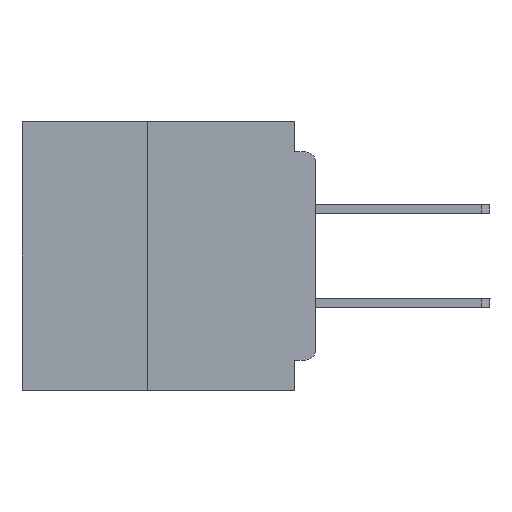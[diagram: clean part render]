
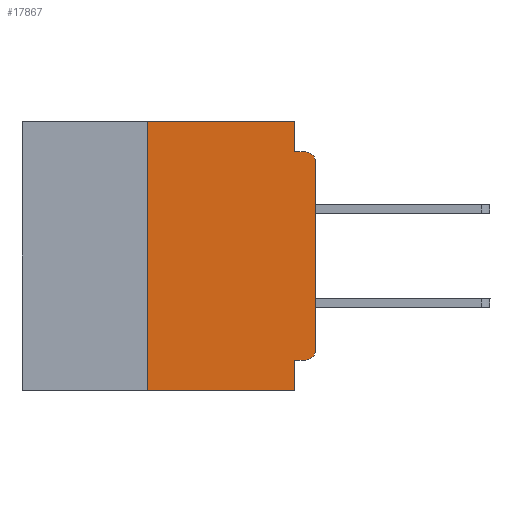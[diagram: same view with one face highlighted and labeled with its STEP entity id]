
A CAD part, left-side view. The second image highlights one B-rep face of the part: STEP entity #17867.
In plain terms, the highlighted planar face has unit normal (-1, 0, 0).
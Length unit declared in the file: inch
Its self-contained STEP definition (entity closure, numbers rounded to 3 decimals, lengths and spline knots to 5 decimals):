
#1379 = VECTOR ( 'NONE', #47287, 39.37008 ) ;
#3993 = CARTESIAN_POINT ( 'NONE',  ( 0., 0., 0. ) ) ;
#5181 = LINE ( 'NONE', #22048, #29538 ) ;
#7249 = VERTEX_POINT ( 'NONE', #17080 ) ;
#7311 = ORIENTED_EDGE ( 'NONE', *, *, #21296, .F. ) ;
#8545 = VERTEX_POINT ( 'NONE', #12974 ) ;
#9433 = VERTEX_POINT ( 'NONE', #9885 ) ;
#9720 = CARTESIAN_POINT ( 'NONE',  ( 0., 0.031, -0.355 ) ) ;
#9763 = ORIENTED_EDGE ( 'NONE', *, *, #60409, .T. ) ;
#9885 = CARTESIAN_POINT ( 'NONE',  ( 0., 0.031, -0.045 ) ) ;
#11398 = CARTESIAN_POINT ( 'NONE',  ( 0., 0., -0.34 ) ) ;
#12096 = DIRECTION ( 'NONE',  ( 0., -1., 0. ) ) ;
#12740 = CARTESIAN_POINT ( 'NONE',  ( 0., 0.031, 0. ) ) ;
#12939 = DIRECTION ( 'NONE',  ( -1., 0., 0. ) ) ;
#12974 = CARTESIAN_POINT ( 'NONE',  ( 0., 0.031, -0.4 ) ) ;
#13891 = VERTEX_POINT ( 'NONE', #11398 ) ;
#13942 = EDGE_CURVE ( 'NONE', #17463, #8545, #29659, .T. ) ;
#14390 = LINE ( 'NONE', #51946, #1379 ) ;
#16096 = PLANE ( 'NONE',  #57764 ) ;
#16668 = CARTESIAN_POINT ( 'NONE',  ( 0., 0.437, -0.4 ) ) ;
#17066 = CARTESIAN_POINT ( 'NONE',  ( 0., 0.015, -0.34 ) ) ;
#17080 = CARTESIAN_POINT ( 'NONE',  ( 0., 0.25, 0. ) ) ;
#17463 = VERTEX_POINT ( 'NONE', #61303 ) ;
#17867 = ADVANCED_FACE ( 'NONE', ( #32133 ), #16096, .F. ) ;
#17999 = DIRECTION ( 'NONE',  ( 0., 0., -1. ) ) ;
#18457 = CARTESIAN_POINT ( 'NONE',  ( 0., 0., -0.06 ) ) ;
#20555 = DIRECTION ( 'NONE',  ( 0., 1., 0. ) ) ;
#21004 = DIRECTION ( 'NONE',  ( 1., 0., 0. ) ) ;
#21126 = CARTESIAN_POINT ( 'NONE',  ( 0., 0.437, 0. ) ) ;
#21296 = EDGE_CURVE ( 'NONE', #9433, #58967, #5181, .T. ) ;
#21410 = CARTESIAN_POINT ( 'NONE',  ( 0., 0.031, 0. ) ) ;
#21971 = DIRECTION ( 'NONE',  ( 0., 0., -1. ) ) ;
#22023 = CARTESIAN_POINT ( 'NONE',  ( 0., 0.015, -0.045 ) ) ;
#22048 = CARTESIAN_POINT ( 'NONE',  ( 0., 0., -0.045 ) ) ;
#22073 = LINE ( 'NONE', #49664, #34943 ) ;
#23579 = DIRECTION ( 'NONE',  ( 0., 0., 1. ) ) ;
#24975 = EDGE_CURVE ( 'NONE', #13891, #28326, #59267, .T. ) ;
#25070 = AXIS2_PLACEMENT_3D ( 'NONE', #41907, #12939, #46710 ) ;
#25267 = ORIENTED_EDGE ( 'NONE', *, *, #54129, .F. ) ;
#25275 = EDGE_CURVE ( 'NONE', #17463, #7249, #29861, .T. ) ;
#26512 = LINE ( 'NONE', #21126, #28064 ) ;
#27000 = CIRCLE ( 'NONE', #34608, 0.015 ) ;
#28064 = VECTOR ( 'NONE', #54672, 39.37008 ) ;
#28326 = VERTEX_POINT ( 'NONE', #18457 ) ;
#28360 = VECTOR ( 'NONE', #31373, 39.37008 ) ;
#28776 = VECTOR ( 'NONE', #17999, 39.37008 ) ;
#28981 = VERTEX_POINT ( 'NONE', #9720 ) ;
#29202 = EDGE_CURVE ( 'NONE', #7249, #40578, #26512, .T. ) ;
#29538 = VECTOR ( 'NONE', #12096, 39.37008 ) ;
#29659 = LINE ( 'NONE', #16668, #40980 ) ;
#29861 = LINE ( 'NONE', #36231, #28360 ) ;
#30119 = CARTESIAN_POINT ( 'NONE',  ( 0., 0.437, 0. ) ) ;
#31373 = DIRECTION ( 'NONE',  ( 0., 0., 1. ) ) ;
#32133 = FACE_OUTER_BOUND ( 'NONE', #49446, .T. ) ;
#34608 = AXIS2_PLACEMENT_3D ( 'NONE', #17066, #50863, #21971 ) ;
#34943 = VECTOR ( 'NONE', #20555, 39.37008 ) ;
#35017 = ORIENTED_EDGE ( 'NONE', *, *, #58791, .F. ) ;
#36231 = CARTESIAN_POINT ( 'NONE',  ( 0., 0.25, -0.4 ) ) ;
#36947 = ORIENTED_EDGE ( 'NONE', *, *, #45676, .F. ) ;
#37871 = VERTEX_POINT ( 'NONE', #45375 ) ;
#40578 = VERTEX_POINT ( 'NONE', #21410 ) ;
#40980 = VECTOR ( 'NONE', #55520, 39.37008 ) ;
#41620 = LINE ( 'NONE', #12740, #28776 ) ;
#41907 = CARTESIAN_POINT ( 'NONE',  ( 0., 0.015, -0.06 ) ) ;
#43517 = ORIENTED_EDGE ( 'NONE', *, *, #25275, .F. ) ;
#43792 = CIRCLE ( 'NONE', #25070, 0.015 ) ;
#45375 = CARTESIAN_POINT ( 'NONE',  ( 0., 0.015, -0.355 ) ) ;
#45676 = EDGE_CURVE ( 'NONE', #40578, #9433, #41620, .T. ) ;
#46470 = VECTOR ( 'NONE', #23579, 39.37008 ) ;
#46710 = DIRECTION ( 'NONE',  ( 0., 0., -1. ) ) ;
#47287 = DIRECTION ( 'NONE',  ( 0., 0., -1. ) ) ;
#49446 = EDGE_LOOP ( 'NONE', ( #52942, #9763, #7311, #36947, #50621, #43517, #53396, #25267, #35017, #55917 ) ) ;
#49664 = CARTESIAN_POINT ( 'NONE',  ( 0., 0., -0.355 ) ) ;
#50621 = ORIENTED_EDGE ( 'NONE', *, *, #29202, .F. ) ;
#50863 = DIRECTION ( 'NONE',  ( -1., 0., 0. ) ) ;
#51946 = CARTESIAN_POINT ( 'NONE',  ( 0., 0.031, -0.4 ) ) ;
#52942 = ORIENTED_EDGE ( 'NONE', *, *, #24975, .T. ) ;
#53396 = ORIENTED_EDGE ( 'NONE', *, *, #13942, .T. ) ;
#54129 = EDGE_CURVE ( 'NONE', #28981, #8545, #14390, .T. ) ;
#54672 = DIRECTION ( 'NONE',  ( 0., -1., 0. ) ) ;
#54754 = DIRECTION ( 'NONE',  ( 0., 0., -1. ) ) ;
#55520 = DIRECTION ( 'NONE',  ( 0., -1., 0. ) ) ;
#55917 = ORIENTED_EDGE ( 'NONE', *, *, #55924, .T. ) ;
#55924 = EDGE_CURVE ( 'NONE', #37871, #13891, #27000, .T. ) ;
#57764 = AXIS2_PLACEMENT_3D ( 'NONE', #30119, #21004, #54754 ) ;
#58791 = EDGE_CURVE ( 'NONE', #37871, #28981, #22073, .T. ) ;
#58967 = VERTEX_POINT ( 'NONE', #22023 ) ;
#59267 = LINE ( 'NONE', #3993, #46470 ) ;
#60409 = EDGE_CURVE ( 'NONE', #28326, #58967, #43792, .T. ) ;
#61303 = CARTESIAN_POINT ( 'NONE',  ( 0., 0.25, -0.4 ) ) ;
